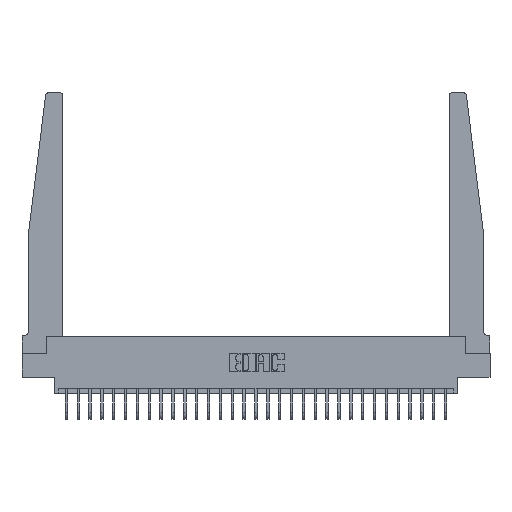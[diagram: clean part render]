
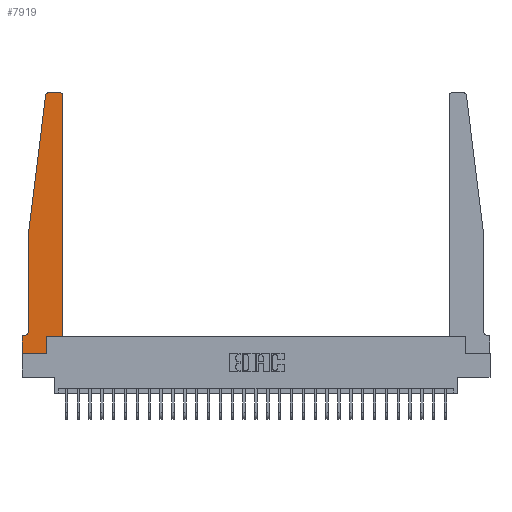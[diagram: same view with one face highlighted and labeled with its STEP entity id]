
A CAD part, top view. The second image highlights one B-rep face of the part: STEP entity #7919.
In plain terms, the highlighted planar face has unit normal (0, 0, 1).
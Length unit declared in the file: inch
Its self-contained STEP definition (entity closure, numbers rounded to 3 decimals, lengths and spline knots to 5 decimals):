
#158 = CARTESIAN_POINT ( 'NONE',  ( 0.395, 2.75, 0.37 ) ) ;
#264 = ORIENTED_EDGE ( 'NONE', *, *, #22088, .T. ) ;
#285 = EDGE_CURVE ( 'NONE', #5303, #14063, #13197, .T. ) ;
#1281 = EDGE_CURVE ( 'NONE', #11683, #20548, #24640, .T. ) ;
#1723 = VERTEX_POINT ( 'NONE', #4069 ) ;
#1771 = VERTEX_POINT ( 'NONE', #6297 ) ;
#2417 = VERTEX_POINT ( 'NONE', #14454 ) ;
#2580 = LINE ( 'NONE', #11338, #8836 ) ;
#2592 = DIRECTION ( 'NONE',  ( -0.122, -0.992, 0. ) ) ;
#2649 = CARTESIAN_POINT ( 'NONE',  ( 0.065, 1.25, 0.37 ) ) ;
#2784 = DIRECTION ( 'NONE',  ( 0., 1., 0. ) ) ;
#2793 = CARTESIAN_POINT ( 'NONE',  ( 0.2605, 0.18, 0.37 ) ) ;
#2928 = AXIS2_PLACEMENT_3D ( 'NONE', #12238, #26498, #14305 ) ;
#3057 = ORIENTED_EDGE ( 'NONE', *, *, #1281, .T. ) ;
#3135 = CARTESIAN_POINT ( 'NONE',  ( 0.065, 1.25, 0.37 ) ) ;
#3137 = CARTESIAN_POINT ( 'NONE',  ( 0.425, 0.18, 0.37 ) ) ;
#3441 = LINE ( 'NONE', #14413, #24030 ) ;
#3847 = VECTOR ( 'NONE', #12318, 39.37008 ) ;
#4069 = CARTESIAN_POINT ( 'NONE',  ( 0.425, 2.72, 0.37 ) ) ;
#4125 = CARTESIAN_POINT ( 'NONE',  ( 0., 0.1875, 0.37 ) ) ;
#4438 = CARTESIAN_POINT ( 'NONE',  ( 0., 0., 0.37 ) ) ;
#5031 = LINE ( 'NONE', #3137, #25548 ) ;
#5110 = PLANE ( 'NONE',  #20490 ) ;
#5202 = EDGE_LOOP ( 'NONE', ( #18538, #14546, #16794, #20849, #11089, #3057, #23229, #10553, #18055, #25945, #264, #6044 ) ) ;
#5211 = CARTESIAN_POINT ( 'NONE',  ( 0., 0.1875, 0.37 ) ) ;
#5303 = VERTEX_POINT ( 'NONE', #17243 ) ;
#6044 = ORIENTED_EDGE ( 'NONE', *, *, #10628, .T. ) ;
#6297 = CARTESIAN_POINT ( 'NONE',  ( 0.065, 0.2375, 0.37 ) ) ;
#7119 = CIRCLE ( 'NONE', #19171, 0.03 ) ;
#7308 = DIRECTION ( 'NONE',  ( 1., 0., 0. ) ) ;
#7566 = FACE_OUTER_BOUND ( 'NONE', #5202, .T. ) ;
#7919 = ADVANCED_FACE ( 'NONE', ( #7566 ), #5110, .T. ) ;
#8111 = CIRCLE ( 'NONE', #18777, 0.05 ) ;
#8243 = CARTESIAN_POINT ( 'NONE',  ( 0.395, 2.72, 0.37 ) ) ;
#8711 = CIRCLE ( 'NONE', #2928, 0.03 ) ;
#8836 = VECTOR ( 'NONE', #23580, 39.37008 ) ;
#9082 = EDGE_CURVE ( 'NONE', #12828, #2417, #2580, .T. ) ;
#9229 = EDGE_CURVE ( 'NONE', #18914, #15458, #20637, .T. ) ;
#9956 = CARTESIAN_POINT ( 'NONE',  ( 0.015, 0.2375, 0.37 ) ) ;
#10160 = VECTOR ( 'NONE', #19548, 39.37008 ) ;
#10297 = DIRECTION ( 'NONE',  ( 1., 0., 0. ) ) ;
#10372 = DIRECTION ( 'NONE',  ( 1., 0., 0. ) ) ;
#10437 = LINE ( 'NONE', #13136, #15260 ) ;
#10553 = ORIENTED_EDGE ( 'NONE', *, *, #9082, .T. ) ;
#10622 = VERTEX_POINT ( 'NONE', #14337 ) ;
#10628 = EDGE_CURVE ( 'NONE', #1723, #18914, #7119, .T. ) ;
#10803 = LINE ( 'NONE', #3135, #10160 ) ;
#10911 = CARTESIAN_POINT ( 'NONE',  ( 0.065, 0.1875, 0.37 ) ) ;
#10914 = VERTEX_POINT ( 'NONE', #2793 ) ;
#11089 = ORIENTED_EDGE ( 'NONE', *, *, #19170, .T. ) ;
#11214 = CARTESIAN_POINT ( 'NONE',  ( 0.27653, 2.75, 0.37 ) ) ;
#11248 = EDGE_CURVE ( 'NONE', #15458, #5303, #8711, .T. ) ;
#11338 = CARTESIAN_POINT ( 'NONE',  ( 0., 0., 0.37 ) ) ;
#11496 = DIRECTION ( 'NONE',  ( 0., 1., 0. ) ) ;
#11683 = VERTEX_POINT ( 'NONE', #19452 ) ;
#12021 = DIRECTION ( 'NONE',  ( -1., 0., 0. ) ) ;
#12238 = CARTESIAN_POINT ( 'NONE',  ( 0.27653, 2.72, 0.37 ) ) ;
#12318 = DIRECTION ( 'NONE',  ( 0., -1., 0. ) ) ;
#12828 = VERTEX_POINT ( 'NONE', #4438 ) ;
#13004 = EDGE_CURVE ( 'NONE', #14063, #1771, #10803, .T. ) ;
#13136 = CARTESIAN_POINT ( 'NONE',  ( 0.2605, 0.18, 0.37 ) ) ;
#13197 = LINE ( 'NONE', #2649, #18658 ) ;
#14063 = VERTEX_POINT ( 'NONE', #18881 ) ;
#14305 = DIRECTION ( 'NONE',  ( 1., 0., 0. ) ) ;
#14337 = CARTESIAN_POINT ( 'NONE',  ( 0.425, 0.18, 0.37 ) ) ;
#14413 = CARTESIAN_POINT ( 'NONE',  ( 0.425, 0.18, 0.37 ) ) ;
#14454 = CARTESIAN_POINT ( 'NONE',  ( 0.2605, 0., 0.37 ) ) ;
#14546 = ORIENTED_EDGE ( 'NONE', *, *, #11248, .T. ) ;
#14873 = LINE ( 'NONE', #18504, #3847 ) ;
#15260 = VECTOR ( 'NONE', #2784, 39.37008 ) ;
#15458 = VERTEX_POINT ( 'NONE', #11214 ) ;
#15889 = VECTOR ( 'NONE', #17895, 39.37008 ) ;
#15934 = CARTESIAN_POINT ( 'NONE',  ( 0.25, 2.75, 0.37 ) ) ;
#16423 = EDGE_CURVE ( 'NONE', #10914, #10622, #3441, .T. ) ;
#16794 = ORIENTED_EDGE ( 'NONE', *, *, #285, .T. ) ;
#17243 = CARTESIAN_POINT ( 'NONE',  ( 0.24675, 2.72367, 0.37 ) ) ;
#17895 = DIRECTION ( 'NONE',  ( -1., 0., 0. ) ) ;
#17968 = VECTOR ( 'NONE', #19138, 39.37008 ) ;
#18055 = ORIENTED_EDGE ( 'NONE', *, *, #23936, .T. ) ;
#18504 = CARTESIAN_POINT ( 'NONE',  ( 0., 0., 0.37 ) ) ;
#18538 = ORIENTED_EDGE ( 'NONE', *, *, #9229, .T. ) ;
#18658 = VECTOR ( 'NONE', #2592, 39.37008 ) ;
#18682 = EDGE_CURVE ( 'NONE', #20548, #12828, #14873, .T. ) ;
#18777 = AXIS2_PLACEMENT_3D ( 'NONE', #9956, #24239, #12021 ) ;
#18881 = CARTESIAN_POINT ( 'NONE',  ( 0.065, 1.25, 0.37 ) ) ;
#18914 = VERTEX_POINT ( 'NONE', #158 ) ;
#19138 = DIRECTION ( 'NONE',  ( -1., 0., 0. ) ) ;
#19170 = EDGE_CURVE ( 'NONE', #1771, #11683, #8111, .T. ) ;
#19171 = AXIS2_PLACEMENT_3D ( 'NONE', #8243, #22531, #10297 ) ;
#19452 = CARTESIAN_POINT ( 'NONE',  ( 0.015, 0.1875, 0.37 ) ) ;
#19548 = DIRECTION ( 'NONE',  ( 0., -1., 0. ) ) ;
#19570 = DIRECTION ( 'NONE',  ( 0., 0., 1. ) ) ;
#20490 = AXIS2_PLACEMENT_3D ( 'NONE', #5211, #19570, #7308 ) ;
#20548 = VERTEX_POINT ( 'NONE', #4125 ) ;
#20637 = LINE ( 'NONE', #15934, #15889 ) ;
#20849 = ORIENTED_EDGE ( 'NONE', *, *, #13004, .T. ) ;
#22088 = EDGE_CURVE ( 'NONE', #10622, #1723, #5031, .T. ) ;
#22531 = DIRECTION ( 'NONE',  ( 0., 0., 1. ) ) ;
#23229 = ORIENTED_EDGE ( 'NONE', *, *, #18682, .T. ) ;
#23580 = DIRECTION ( 'NONE',  ( 1., 0., 0. ) ) ;
#23936 = EDGE_CURVE ( 'NONE', #2417, #10914, #10437, .T. ) ;
#24030 = VECTOR ( 'NONE', #10372, 39.37008 ) ;
#24239 = DIRECTION ( 'NONE',  ( 0., 0., -1. ) ) ;
#24640 = LINE ( 'NONE', #10911, #17968 ) ;
#25548 = VECTOR ( 'NONE', #11496, 39.37008 ) ;
#25945 = ORIENTED_EDGE ( 'NONE', *, *, #16423, .T. ) ;
#26498 = DIRECTION ( 'NONE',  ( 0., 0., 1. ) ) ;
